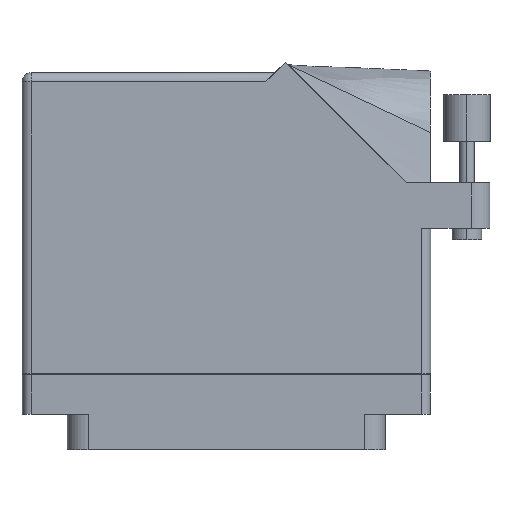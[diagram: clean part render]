
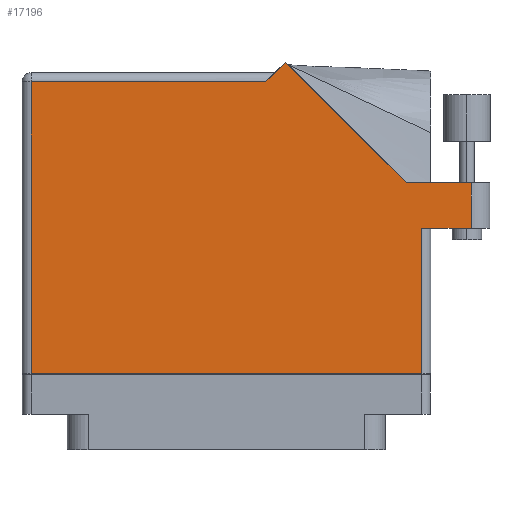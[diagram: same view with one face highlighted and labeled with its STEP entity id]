
A CAD part, front view. The second image highlights one B-rep face of the part: STEP entity #17196.
In plain terms, the highlighted face is planar.
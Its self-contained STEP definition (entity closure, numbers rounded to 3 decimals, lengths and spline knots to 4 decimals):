
#159 = CARTESIAN_POINT ( 'NONE',  ( 1.7775, 1.187, 0.765 ) ) ;
#2506 = LINE ( 'NONE', #159, #20540 ) ;
#2541 = ORIENTED_EDGE ( 'NONE', *, *, #22253, .T. ) ;
#2920 = ORIENTED_EDGE ( 'NONE', *, *, #36971, .T. ) ;
#3178 = ORIENTED_EDGE ( 'NONE', *, *, #66893, .T. ) ;
#4722 = VERTEX_POINT ( 'NONE', #26017 ) ;
#7637 = DIRECTION ( 'NONE',  ( -0.707, -0.707, 0. ) ) ;
#8145 = VERTEX_POINT ( 'NONE', #47654 ) ;
#9699 = EDGE_CURVE ( 'NONE', #59850, #68838, #76688, .T. ) ;
#10422 = CARTESIAN_POINT ( 'NONE',  ( -1.3775, 1.93, 0.765 ) ) ;
#11340 = DIRECTION ( 'NONE',  ( -0.707, 0.707, 0. ) ) ;
#11701 = VECTOR ( 'NONE', #11340, 39.3701 ) ;
#12095 = CARTESIAN_POINT ( 'NONE',  ( -1.3155, -0.1, 0.765 ) ) ;
#15854 = EDGE_CURVE ( 'NONE', #36383, #4722, #73818, .T. ) ;
#15981 = ORIENTED_EDGE ( 'NONE', *, *, #15854, .T. ) ;
#16047 = CARTESIAN_POINT ( 'NONE',  ( 1.6525, 1.187, 0.765 ) ) ;
#17196 = ADVANCED_FACE ( 'NONE', ( #55694 ), #54238, .F. ) ;
#20540 = VECTOR ( 'NONE', #25891, 39.3701 ) ;
#20826 = ORIENTED_EDGE ( 'NONE', *, *, #56835, .T. ) ;
#21270 = ORIENTED_EDGE ( 'NONE', *, *, #9699, .T. ) ;
#21544 = LINE ( 'NONE', #12095, #59468 ) ;
#22253 = EDGE_CURVE ( 'NONE', #68838, #8145, #81028, .T. ) ;
#25648 = ORIENTED_EDGE ( 'NONE', *, *, #44061, .T. ) ;
#25891 = DIRECTION ( 'NONE',  ( -1., 0., 0. ) ) ;
#26017 = CARTESIAN_POINT ( 'NONE',  ( 1.6525, 1.187, 0.765 ) ) ;
#28793 = CARTESIAN_POINT ( 'NONE',  ( 0.2655, 1.868, 0.765 ) ) ;
#30740 = CARTESIAN_POINT ( 'NONE',  ( 1.3775, 0.88, 0.765 ) ) ;
#32163 = EDGE_CURVE ( 'NONE', #52051, #36383, #38284, .T. ) ;
#35520 = DIRECTION ( 'NONE',  ( 0., 0., -1. ) ) ;
#36052 = CARTESIAN_POINT ( 'NONE',  ( 0.3982, 2.0007, 0.765 ) ) ;
#36315 = CARTESIAN_POINT ( 'NONE',  ( -1.3155, -0.1, 0.765 ) ) ;
#36383 = VERTEX_POINT ( 'NONE', #40826 ) ;
#36626 = CARTESIAN_POINT ( 'NONE',  ( -1.3775, -0.1, 0.765 ) ) ;
#36971 = EDGE_CURVE ( 'NONE', #4722, #50369, #2506, .T. ) ;
#37483 = ORIENTED_EDGE ( 'NONE', *, *, #32163, .T. ) ;
#38284 = LINE ( 'NONE', #30740, #53290 ) ;
#38359 = CARTESIAN_POINT ( 'NONE',  ( 1.3155, -0.1, 0.765 ) ) ;
#40722 = VECTOR ( 'NONE', #7637, 39.3701 ) ;
#40826 = CARTESIAN_POINT ( 'NONE',  ( 1.6525, 0.88, 0.765 ) ) ;
#44061 = EDGE_CURVE ( 'NONE', #56345, #45064, #63108, .T. ) ;
#44380 = CARTESIAN_POINT ( 'NONE',  ( 1.3155, 0.88, 0.765 ) ) ;
#44470 = DIRECTION ( 'NONE',  ( 0., -1., 0. ) ) ;
#45064 = VERTEX_POINT ( 'NONE', #38359 ) ;
#46165 = VECTOR ( 'NONE', #49736, 39.3701 ) ;
#46399 = EDGE_CURVE ( 'NONE', #45064, #52051, #74470, .T. ) ;
#47654 = CARTESIAN_POINT ( 'NONE',  ( -1.3155, 1.868, 0.765 ) ) ;
#49467 = VECTOR ( 'NONE', #63293, 39.3701 ) ;
#49736 = DIRECTION ( 'NONE',  ( 1., 0., 0. ) ) ;
#50369 = VERTEX_POINT ( 'NONE', #80016 ) ;
#50870 = CARTESIAN_POINT ( 'NONE',  ( 1.3155, 0.88, 0.765 ) ) ;
#52051 = VERTEX_POINT ( 'NONE', #50870 ) ;
#53089 = AXIS2_PLACEMENT_3D ( 'NONE', #10422, #35520, #67892 ) ;
#53290 = VECTOR ( 'NONE', #56371, 39.3701 ) ;
#53999 = DIRECTION ( 'NONE',  ( 0., 1., 0. ) ) ;
#54238 = PLANE ( 'NONE',  #53089 ) ;
#55694 = FACE_OUTER_BOUND ( 'NONE', #73396, .T. ) ;
#56345 = VERTEX_POINT ( 'NONE', #36315 ) ;
#56371 = DIRECTION ( 'NONE',  ( 1., 0., 0. ) ) ;
#56784 = VECTOR ( 'NONE', #53999, 39.3701 ) ;
#56835 = EDGE_CURVE ( 'NONE', #50369, #59850, #68652, .T. ) ;
#57953 = DIRECTION ( 'NONE',  ( -1., 0., 0. ) ) ;
#57976 = VECTOR ( 'NONE', #57953, 39.3701 ) ;
#58413 = CARTESIAN_POINT ( 'NONE',  ( 0.3275, 1.93, 0.765 ) ) ;
#59468 = VECTOR ( 'NONE', #44470, 39.3701 ) ;
#59850 = VERTEX_POINT ( 'NONE', #36052 ) ;
#60802 = ORIENTED_EDGE ( 'NONE', *, *, #46399, .T. ) ;
#63108 = LINE ( 'NONE', #36626, #46165 ) ;
#63293 = DIRECTION ( 'NONE',  ( 0., 1., 0. ) ) ;
#65176 = CARTESIAN_POINT ( 'NONE',  ( -1.3775, 1.868, 0.765 ) ) ;
#66893 = EDGE_CURVE ( 'NONE', #8145, #56345, #21544, .T. ) ;
#67892 = DIRECTION ( 'NONE',  ( -1., 0., 0. ) ) ;
#68652 = LINE ( 'NONE', #80011, #11701 ) ;
#68838 = VERTEX_POINT ( 'NONE', #28793 ) ;
#73396 = EDGE_LOOP ( 'NONE', ( #37483, #15981, #2920, #20826, #21270, #2541, #3178, #25648, #60802 ) ) ;
#73818 = LINE ( 'NONE', #16047, #56784 ) ;
#74470 = LINE ( 'NONE', #44380, #49467 ) ;
#76688 = LINE ( 'NONE', #58413, #40722 ) ;
#80011 = CARTESIAN_POINT ( 'NONE',  ( 1.2119, 1.187, 0.765 ) ) ;
#80016 = CARTESIAN_POINT ( 'NONE',  ( 1.2119, 1.187, 0.765 ) ) ;
#81028 = LINE ( 'NONE', #65176, #57976 ) ;
